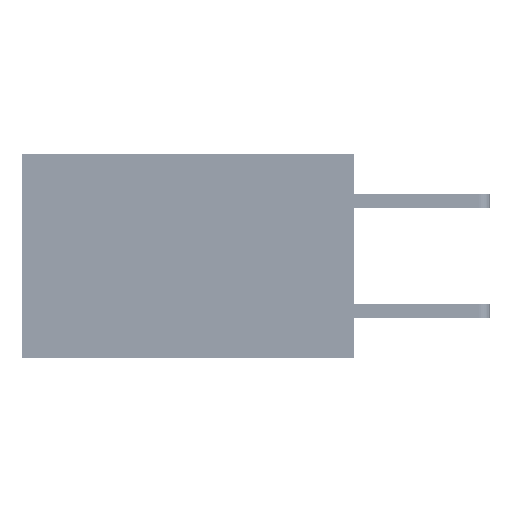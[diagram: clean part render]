
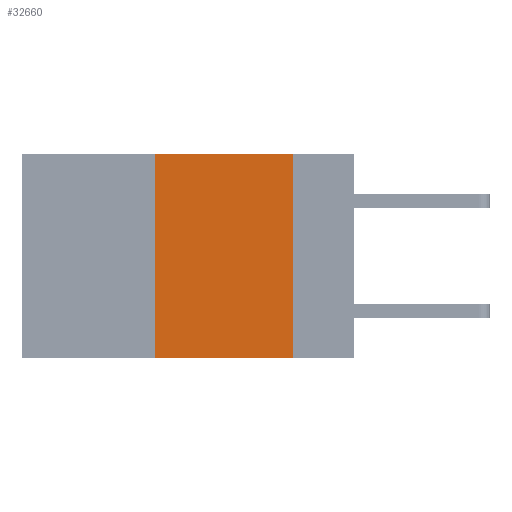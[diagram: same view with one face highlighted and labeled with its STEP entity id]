
A CAD part, left-side view. The second image highlights one B-rep face of the part: STEP entity #32660.
In plain terms, the highlighted planar face has unit normal (-1, 0, 0).
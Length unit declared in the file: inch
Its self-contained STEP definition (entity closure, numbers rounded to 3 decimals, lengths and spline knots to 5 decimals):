
#1038 = CARTESIAN_POINT ( 'NONE',  ( 0., 0.6, -0.37 ) ) ;
#1600 = VERTEX_POINT ( 'NONE', #26154 ) ;
#2115 = CARTESIAN_POINT ( 'NONE',  ( 0., 0.11, 0. ) ) ;
#3490 = CARTESIAN_POINT ( 'NONE',  ( 0., 0.11, 0. ) ) ;
#4973 = DIRECTION ( 'NONE',  ( 1., 0., 0. ) ) ;
#8402 = LINE ( 'NONE', #11546, #31295 ) ;
#8762 = EDGE_CURVE ( 'NONE', #25625, #25501, #11928, .T. ) ;
#9092 = EDGE_LOOP ( 'NONE', ( #18400, #27943, #11885, #10788 ) ) ;
#10614 = EDGE_CURVE ( 'NONE', #1600, #14710, #8402, .T. ) ;
#10788 = ORIENTED_EDGE ( 'NONE', *, *, #27925, .T. ) ;
#11546 = CARTESIAN_POINT ( 'NONE',  ( 0., 0.36, 0. ) ) ;
#11885 = ORIENTED_EDGE ( 'NONE', *, *, #10614, .F. ) ;
#11928 = LINE ( 'NONE', #2115, #35200 ) ;
#14402 = AXIS2_PLACEMENT_3D ( 'NONE', #30653, #4973, #24395 ) ;
#14710 = VERTEX_POINT ( 'NONE', #26260 ) ;
#18145 = FACE_OUTER_BOUND ( 'NONE', #9092, .T. ) ;
#18400 = ORIENTED_EDGE ( 'NONE', *, *, #8762, .F. ) ;
#20928 = DIRECTION ( 'NONE',  ( 0., 0., -1. ) ) ;
#23168 = VECTOR ( 'NONE', #29598, 39.37008 ) ;
#24290 = DIRECTION ( 'NONE',  ( 0., 0., 1. ) ) ;
#24395 = DIRECTION ( 'NONE',  ( 0., 0., -1. ) ) ;
#25501 = VERTEX_POINT ( 'NONE', #40679 ) ;
#25594 = EDGE_CURVE ( 'NONE', #14710, #25625, #29392, .T. ) ;
#25625 = VERTEX_POINT ( 'NONE', #3490 ) ;
#25916 = DIRECTION ( 'NONE',  ( 0., -1., 0. ) ) ;
#26154 = CARTESIAN_POINT ( 'NONE',  ( 0., 0.36, -0.37 ) ) ;
#26260 = CARTESIAN_POINT ( 'NONE',  ( 0., 0.36, 0. ) ) ;
#26665 = CARTESIAN_POINT ( 'NONE',  ( 0., 0.6, 0. ) ) ;
#27925 = EDGE_CURVE ( 'NONE', #1600, #25501, #39476, .T. ) ;
#27943 = ORIENTED_EDGE ( 'NONE', *, *, #25594, .F. ) ;
#29392 = LINE ( 'NONE', #26665, #23168 ) ;
#29598 = DIRECTION ( 'NONE',  ( 0., -1., 0. ) ) ;
#30653 = CARTESIAN_POINT ( 'NONE',  ( 0., 0.6, 0. ) ) ;
#30866 = PLANE ( 'NONE',  #14402 ) ;
#31295 = VECTOR ( 'NONE', #24290, 39.37008 ) ;
#32660 = ADVANCED_FACE ( 'NONE', ( #18145 ), #30866, .F. ) ;
#34637 = VECTOR ( 'NONE', #25916, 39.37008 ) ;
#35200 = VECTOR ( 'NONE', #20928, 39.37008 ) ;
#39476 = LINE ( 'NONE', #1038, #34637 ) ;
#40679 = CARTESIAN_POINT ( 'NONE',  ( 0., 0.11, -0.37 ) ) ;
